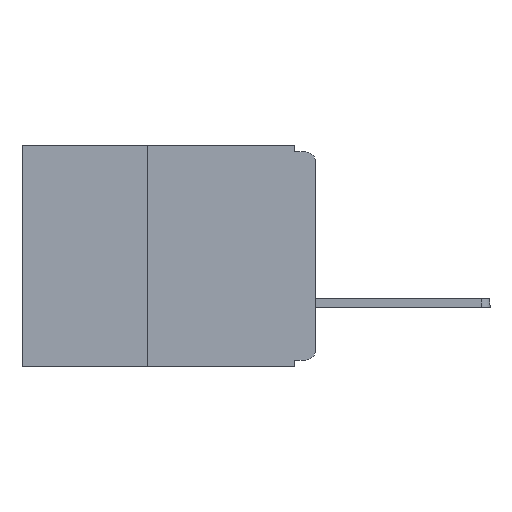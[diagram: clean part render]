
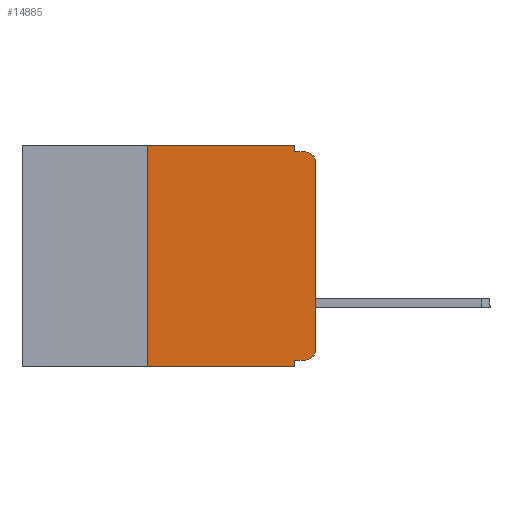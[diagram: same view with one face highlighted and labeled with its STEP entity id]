
A CAD part, left-side view. The second image highlights one B-rep face of the part: STEP entity #14885.
In plain terms, the highlighted planar face has unit normal (-1, 0, 0).
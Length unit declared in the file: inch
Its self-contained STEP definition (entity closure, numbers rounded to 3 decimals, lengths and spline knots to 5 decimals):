
#514 = ORIENTED_EDGE ( 'NONE', *, *, #13506, .F. ) ;
#909 = VERTEX_POINT ( 'NONE', #20480 ) ;
#1099 = CARTESIAN_POINT ( 'NONE',  ( 0., 0.437, -0.33 ) ) ;
#1445 = CARTESIAN_POINT ( 'NONE',  ( 0., 0.031, 0. ) ) ;
#1611 = LINE ( 'NONE', #1099, #16636 ) ;
#1917 = VERTEX_POINT ( 'NONE', #25222 ) ;
#2542 = EDGE_CURVE ( 'NONE', #15719, #1917, #16742, .T. ) ;
#3050 = EDGE_CURVE ( 'NONE', #20538, #15719, #24981, .T. ) ;
#3351 = DIRECTION ( 'NONE',  ( 0., 1., 0. ) ) ;
#3490 = VECTOR ( 'NONE', #13896, 39.37008 ) ;
#4003 = EDGE_LOOP ( 'NONE', ( #5299, #7909, #10490, #25104, #6970, #514, #13994, #13044, #24228, #25505 ) ) ;
#4886 = LINE ( 'NONE', #19200, #15128 ) ;
#4894 = VECTOR ( 'NONE', #3351, 39.37008 ) ;
#5026 = CARTESIAN_POINT ( 'NONE',  ( 0., 0.015, -0.025 ) ) ;
#5299 = ORIENTED_EDGE ( 'NONE', *, *, #2542, .T. ) ;
#6865 = VECTOR ( 'NONE', #23436, 39.37008 ) ;
#6970 = ORIENTED_EDGE ( 'NONE', *, *, #18731, .F. ) ;
#7106 = CARTESIAN_POINT ( 'NONE',  ( 0., 0.031, -0.01 ) ) ;
#7122 = DIRECTION ( 'NONE',  ( 0., 0., -1. ) ) ;
#7693 = LINE ( 'NONE', #26086, #3490 ) ;
#7874 = CARTESIAN_POINT ( 'NONE',  ( 0., 0.437, 0. ) ) ;
#7909 = ORIENTED_EDGE ( 'NONE', *, *, #20096, .T. ) ;
#8383 = VERTEX_POINT ( 'NONE', #7106 ) ;
#8633 = CIRCLE ( 'NONE', #11420, 0.015 ) ;
#8984 = CARTESIAN_POINT ( 'NONE',  ( 0., 0.031, -0.33 ) ) ;
#9097 = DIRECTION ( 'NONE',  ( 0., 0., -1. ) ) ;
#9126 = DIRECTION ( 'NONE',  ( -1., 0., 0. ) ) ;
#9163 = CARTESIAN_POINT ( 'NONE',  ( 0., 0.015, -0.305 ) ) ;
#9631 = VERTEX_POINT ( 'NONE', #17274 ) ;
#9871 = FACE_OUTER_BOUND ( 'NONE', #4003, .T. ) ;
#9981 = VECTOR ( 'NONE', #23686, 39.37008 ) ;
#10490 = ORIENTED_EDGE ( 'NONE', *, *, #22545, .F. ) ;
#10965 = DIRECTION ( 'NONE',  ( 0., 0., -1. ) ) ;
#11413 = EDGE_CURVE ( 'NONE', #909, #13252, #12599, .T. ) ;
#11420 = AXIS2_PLACEMENT_3D ( 'NONE', #5026, #19320, #7122 ) ;
#11975 = DIRECTION ( 'NONE',  ( 0., 0., -1. ) ) ;
#12599 = LINE ( 'NONE', #23141, #18003 ) ;
#12890 = CARTESIAN_POINT ( 'NONE',  ( 0., 0.015, -0.32 ) ) ;
#13044 = ORIENTED_EDGE ( 'NONE', *, *, #11413, .F. ) ;
#13252 = VERTEX_POINT ( 'NONE', #8984 ) ;
#13352 = DIRECTION ( 'NONE',  ( 0., -1., 0. ) ) ;
#13506 = EDGE_CURVE ( 'NONE', #24548, #13881, #7693, .T. ) ;
#13881 = VERTEX_POINT ( 'NONE', #23229 ) ;
#13896 = DIRECTION ( 'NONE',  ( 0., 0., 1. ) ) ;
#13994 = ORIENTED_EDGE ( 'NONE', *, *, #18686, .T. ) ;
#14885 = ADVANCED_FACE ( 'NONE', ( #9871 ), #22102, .F. ) ;
#15128 = VECTOR ( 'NONE', #23301, 39.37008 ) ;
#15328 = AXIS2_PLACEMENT_3D ( 'NONE', #9163, #9126, #9097 ) ;
#15719 = VERTEX_POINT ( 'NONE', #16625 ) ;
#15774 = LINE ( 'NONE', #21657, #4894 ) ;
#16092 = VECTOR ( 'NONE', #20618, 39.37008 ) ;
#16554 = EDGE_CURVE ( 'NONE', #26179, #8383, #23118, .T. ) ;
#16625 = CARTESIAN_POINT ( 'NONE',  ( 0., 0., -0.305 ) ) ;
#16636 = VECTOR ( 'NONE', #13352, 39.37008 ) ;
#16643 = EDGE_CURVE ( 'NONE', #20538, #909, #15774, .T. ) ;
#16742 = LINE ( 'NONE', #20768, #16092 ) ;
#17274 = CARTESIAN_POINT ( 'NONE',  ( 0., 0.015, -0.01 ) ) ;
#17572 = CARTESIAN_POINT ( 'NONE',  ( 0., 0.437, 0. ) ) ;
#18003 = VECTOR ( 'NONE', #10965, 39.37008 ) ;
#18686 = EDGE_CURVE ( 'NONE', #24548, #13252, #1611, .T. ) ;
#18731 = EDGE_CURVE ( 'NONE', #13881, #26179, #22048, .T. ) ;
#19200 = CARTESIAN_POINT ( 'NONE',  ( 0., 0., -0.01 ) ) ;
#19320 = DIRECTION ( 'NONE',  ( -1., 0., 0. ) ) ;
#20096 = EDGE_CURVE ( 'NONE', #1917, #9631, #8633, .T. ) ;
#20480 = CARTESIAN_POINT ( 'NONE',  ( 0., 0.031, -0.32 ) ) ;
#20538 = VERTEX_POINT ( 'NONE', #12890 ) ;
#20618 = DIRECTION ( 'NONE',  ( 0., 0., 1. ) ) ;
#20768 = CARTESIAN_POINT ( 'NONE',  ( 0., 0., 0. ) ) ;
#21384 = CARTESIAN_POINT ( 'NONE',  ( 0., 0.031, 0. ) ) ;
#21657 = CARTESIAN_POINT ( 'NONE',  ( 0., 0., -0.32 ) ) ;
#22048 = LINE ( 'NONE', #17572, #9981 ) ;
#22100 = CARTESIAN_POINT ( 'NONE',  ( 0., 0.25, -0.33 ) ) ;
#22102 = PLANE ( 'NONE',  #26279 ) ;
#22545 = EDGE_CURVE ( 'NONE', #8383, #9631, #4886, .T. ) ;
#23118 = LINE ( 'NONE', #21384, #6865 ) ;
#23141 = CARTESIAN_POINT ( 'NONE',  ( 0., 0.031, -0.33 ) ) ;
#23229 = CARTESIAN_POINT ( 'NONE',  ( 0., 0.25, 0. ) ) ;
#23301 = DIRECTION ( 'NONE',  ( 0., -1., 0. ) ) ;
#23436 = DIRECTION ( 'NONE',  ( 0., 0., -1. ) ) ;
#23686 = DIRECTION ( 'NONE',  ( 0., -1., 0. ) ) ;
#24133 = DIRECTION ( 'NONE',  ( 1., 0., 0. ) ) ;
#24228 = ORIENTED_EDGE ( 'NONE', *, *, #16643, .F. ) ;
#24548 = VERTEX_POINT ( 'NONE', #22100 ) ;
#24981 = CIRCLE ( 'NONE', #15328, 0.015 ) ;
#25104 = ORIENTED_EDGE ( 'NONE', *, *, #16554, .F. ) ;
#25222 = CARTESIAN_POINT ( 'NONE',  ( 0., 0., -0.025 ) ) ;
#25505 = ORIENTED_EDGE ( 'NONE', *, *, #3050, .T. ) ;
#26086 = CARTESIAN_POINT ( 'NONE',  ( 0., 0.25, -0.33 ) ) ;
#26179 = VERTEX_POINT ( 'NONE', #1445 ) ;
#26279 = AXIS2_PLACEMENT_3D ( 'NONE', #7874, #24133, #11975 ) ;
